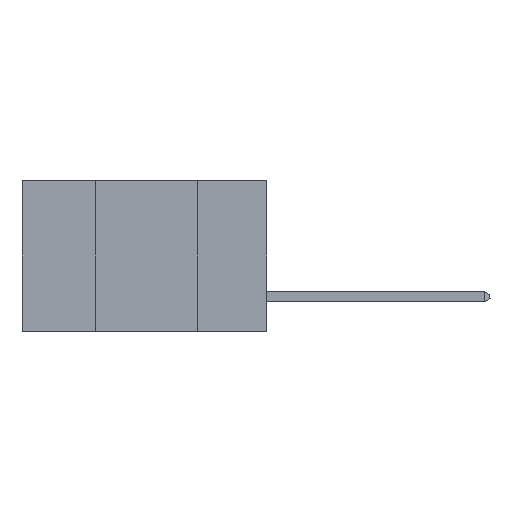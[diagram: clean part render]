
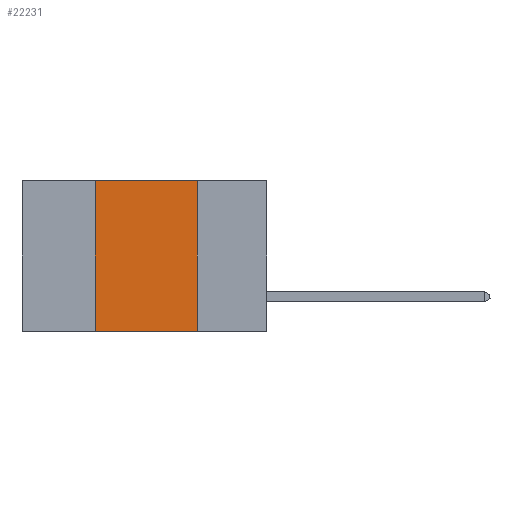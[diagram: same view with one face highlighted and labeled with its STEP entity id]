
A CAD part, left-side view. The second image highlights one B-rep face of the part: STEP entity #22231.
In plain terms, the highlighted planar face has unit normal (-1, 0, 0).
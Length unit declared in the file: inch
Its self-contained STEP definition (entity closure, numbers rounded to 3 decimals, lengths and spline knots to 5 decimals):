
#29 = ORIENTED_EDGE ( 'NONE', *, *, #12617, .T. ) ;
#4651 = EDGE_CURVE ( 'NONE', #7209, #20720, #14234, .T. ) ;
#4933 = DIRECTION ( 'NONE',  ( 0., 0., 1. ) ) ;
#5027 = ORIENTED_EDGE ( 'NONE', *, *, #18419, .F. ) ;
#5198 = LINE ( 'NONE', #11352, #25460 ) ;
#5633 = DIRECTION ( 'NONE',  ( 0., 0., -1. ) ) ;
#5643 = VERTEX_POINT ( 'NONE', #8119 ) ;
#5971 = VECTOR ( 'NONE', #4933, 39.37008 ) ;
#6802 = EDGE_LOOP ( 'NONE', ( #24412, #5027, #25326, #29 ) ) ;
#7102 = LINE ( 'NONE', #13025, #13494 ) ;
#7209 = VERTEX_POINT ( 'NONE', #20674 ) ;
#8119 = CARTESIAN_POINT ( 'NONE',  ( 0., 0.17, -0.37 ) ) ;
#10967 = DIRECTION ( 'NONE',  ( 0., 0., -1. ) ) ;
#11352 = CARTESIAN_POINT ( 'NONE',  ( 0., 0.6, -0.37 ) ) ;
#12617 = EDGE_CURVE ( 'NONE', #7209, #5643, #5198, .T. ) ;
#13025 = CARTESIAN_POINT ( 'NONE',  ( 0., 0.17, 0. ) ) ;
#13494 = VECTOR ( 'NONE', #10967, 39.37008 ) ;
#13961 = VECTOR ( 'NONE', #19493, 39.37008 ) ;
#14234 = LINE ( 'NONE', #15037, #5971 ) ;
#14313 = LINE ( 'NONE', #17298, #13961 ) ;
#14801 = FACE_OUTER_BOUND ( 'NONE', #6802, .T. ) ;
#15010 = EDGE_CURVE ( 'NONE', #24874, #5643, #7102, .T. ) ;
#15037 = CARTESIAN_POINT ( 'NONE',  ( 0., 0.42, 0. ) ) ;
#17298 = CARTESIAN_POINT ( 'NONE',  ( 0., 0.6, 0. ) ) ;
#17859 = DIRECTION ( 'NONE',  ( 1., 0., 0. ) ) ;
#18038 = PLANE ( 'NONE',  #23697 ) ;
#18419 = EDGE_CURVE ( 'NONE', #20720, #24874, #14313, .T. ) ;
#19493 = DIRECTION ( 'NONE',  ( 0., -1., 0. ) ) ;
#19874 = CARTESIAN_POINT ( 'NONE',  ( 0., 0.6, 0. ) ) ;
#20674 = CARTESIAN_POINT ( 'NONE',  ( 0., 0.42, -0.37 ) ) ;
#20720 = VERTEX_POINT ( 'NONE', #23476 ) ;
#21491 = DIRECTION ( 'NONE',  ( 0., -1., 0. ) ) ;
#22231 = ADVANCED_FACE ( 'NONE', ( #14801 ), #18038, .F. ) ;
#23088 = CARTESIAN_POINT ( 'NONE',  ( 0., 0.17, 0. ) ) ;
#23476 = CARTESIAN_POINT ( 'NONE',  ( 0., 0.42, 0. ) ) ;
#23697 = AXIS2_PLACEMENT_3D ( 'NONE', #19874, #17859, #5633 ) ;
#24412 = ORIENTED_EDGE ( 'NONE', *, *, #15010, .F. ) ;
#24874 = VERTEX_POINT ( 'NONE', #23088 ) ;
#25326 = ORIENTED_EDGE ( 'NONE', *, *, #4651, .F. ) ;
#25460 = VECTOR ( 'NONE', #21491, 39.37008 ) ;
